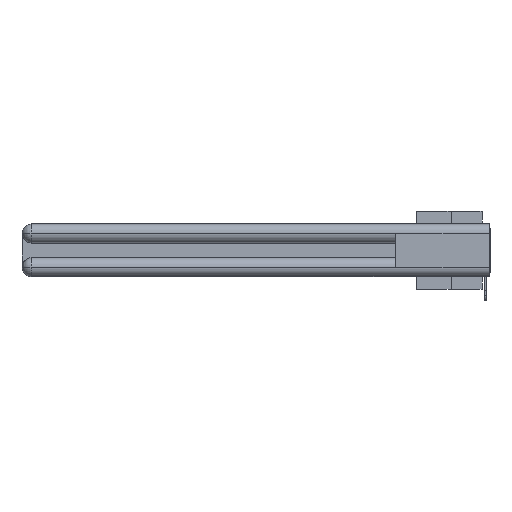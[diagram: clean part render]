
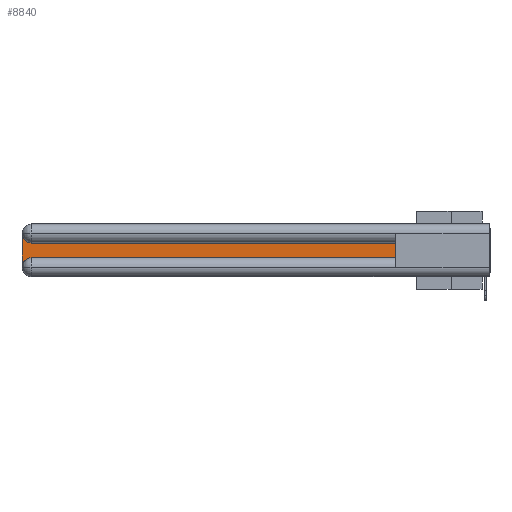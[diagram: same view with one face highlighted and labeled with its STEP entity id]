
A CAD part, left-side view. The second image highlights one B-rep face of the part: STEP entity #8840.
In plain terms, the highlighted planar face has unit normal (-1, 0, 0).
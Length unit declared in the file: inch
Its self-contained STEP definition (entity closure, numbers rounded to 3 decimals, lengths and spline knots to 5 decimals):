
#732 = VECTOR ( 'NONE', #23733, 39.37008 ) ;
#948 = ORIENTED_EDGE ( 'NONE', *, *, #22846, .T. ) ;
#3747 = EDGE_CURVE ( 'NONE', #23247, #34745, #13339, .T. ) ;
#3780 = FACE_OUTER_BOUND ( 'NONE', #7522, .T. ) ;
#4761 = ORIENTED_EDGE ( 'NONE', *, *, #15465, .T. ) ;
#7522 = EDGE_LOOP ( 'NONE', ( #37412, #948, #33932, #32966, #38460, #4761 ) ) ;
#7915 = CARTESIAN_POINT ( 'NONE',  ( 0.075, 3., -0.2175 ) ) ;
#8840 = ADVANCED_FACE ( 'NONE', ( #3780 ), #14611, .F. ) ;
#9814 = LINE ( 'NONE', #18124, #732 ) ;
#10711 = DIRECTION ( 'NONE',  ( 0., 0., -1. ) ) ;
#11551 = DIRECTION ( 'NONE',  ( 0., 0., -1. ) ) ;
#12403 = DIRECTION ( 'NONE',  ( 0., -1., 0. ) ) ;
#13320 = DIRECTION ( 'NONE',  ( 1., 0., 0. ) ) ;
#13339 = LINE ( 'NONE', #36624, #39210 ) ;
#14611 = PLANE ( 'NONE',  #20088 ) ;
#14697 = CARTESIAN_POINT ( 'NONE',  ( 0.075, 3., -0.0625 ) ) ;
#15465 = EDGE_CURVE ( 'NONE', #34745, #26085, #19568, .T. ) ;
#15930 = CARTESIAN_POINT ( 'NONE',  ( 0.075, 0.6, -0.2175 ) ) ;
#16796 = VERTEX_POINT ( 'NONE', #26614 ) ;
#17338 = AXIS2_PLACEMENT_3D ( 'NONE', #35077, #38159, #28784 ) ;
#18124 = CARTESIAN_POINT ( 'NONE',  ( 0.075, 0.6, -0.1225 ) ) ;
#18426 = EDGE_CURVE ( 'NONE', #26085, #29140, #9814, .T. ) ;
#18738 = VECTOR ( 'NONE', #10711, 39.37008 ) ;
#19468 = CARTESIAN_POINT ( 'NONE',  ( 0.075, 2.94, -0.0625 ) ) ;
#19530 = DIRECTION ( 'NONE',  ( 0., 0., 1. ) ) ;
#19568 = LINE ( 'NONE', #15930, #31527 ) ;
#20088 = AXIS2_PLACEMENT_3D ( 'NONE', #23950, #39217, #11551 ) ;
#20313 = EDGE_CURVE ( 'NONE', #29690, #16796, #31167, .T. ) ;
#21735 = CARTESIAN_POINT ( 'NONE',  ( 0.075, 0.6, -0.2175 ) ) ;
#22846 = EDGE_CURVE ( 'NONE', #29140, #29690, #28717, .T. ) ;
#23247 = VERTEX_POINT ( 'NONE', #33076 ) ;
#23733 = DIRECTION ( 'NONE',  ( 0., 1., 0. ) ) ;
#23950 = CARTESIAN_POINT ( 'NONE',  ( 0.075, 3., -0.1225 ) ) ;
#26085 = VERTEX_POINT ( 'NONE', #30527 ) ;
#26411 = EDGE_CURVE ( 'NONE', #16796, #23247, #31510, .T. ) ;
#26614 = CARTESIAN_POINT ( 'NONE',  ( 0.075, 3., -0.2775 ) ) ;
#28717 = CIRCLE ( 'NONE', #37269, 0.06 ) ;
#28784 = DIRECTION ( 'NONE',  ( 0., 0., -1. ) ) ;
#29140 = VERTEX_POINT ( 'NONE', #36296 ) ;
#29690 = VERTEX_POINT ( 'NONE', #14697 ) ;
#30527 = CARTESIAN_POINT ( 'NONE',  ( 0.075, 0.6, -0.1225 ) ) ;
#31167 = LINE ( 'NONE', #7915, #18738 ) ;
#31510 = CIRCLE ( 'NONE', #17338, 0.06 ) ;
#31527 = VECTOR ( 'NONE', #19530, 39.37008 ) ;
#32966 = ORIENTED_EDGE ( 'NONE', *, *, #26411, .T. ) ;
#33076 = CARTESIAN_POINT ( 'NONE',  ( 0.075, 2.94, -0.2175 ) ) ;
#33932 = ORIENTED_EDGE ( 'NONE', *, *, #20313, .T. ) ;
#34714 = DIRECTION ( 'NONE',  ( 0., 0., -1. ) ) ;
#34745 = VERTEX_POINT ( 'NONE', #21735 ) ;
#35077 = CARTESIAN_POINT ( 'NONE',  ( 0.075, 2.94, -0.2775 ) ) ;
#36296 = CARTESIAN_POINT ( 'NONE',  ( 0.075, 2.94, -0.1225 ) ) ;
#36624 = CARTESIAN_POINT ( 'NONE',  ( 0.075, 0.6, -0.2175 ) ) ;
#37269 = AXIS2_PLACEMENT_3D ( 'NONE', #19468, #13320, #34714 ) ;
#37412 = ORIENTED_EDGE ( 'NONE', *, *, #18426, .T. ) ;
#38159 = DIRECTION ( 'NONE',  ( 1., 0., 0. ) ) ;
#38460 = ORIENTED_EDGE ( 'NONE', *, *, #3747, .T. ) ;
#39210 = VECTOR ( 'NONE', #12403, 39.37008 ) ;
#39217 = DIRECTION ( 'NONE',  ( 1., 0., 0. ) ) ;
